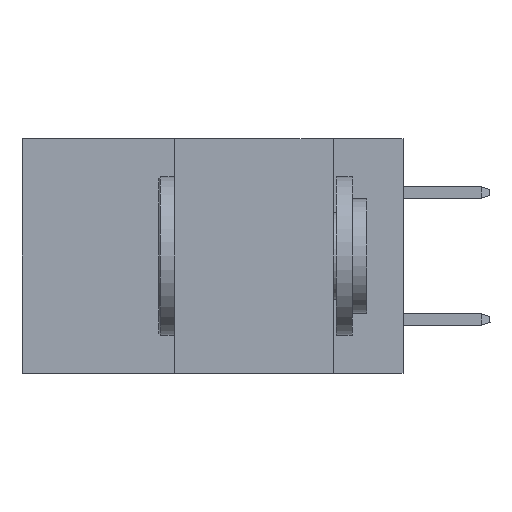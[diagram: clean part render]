
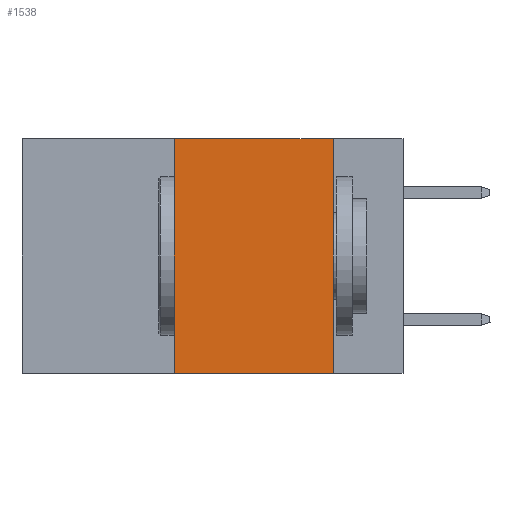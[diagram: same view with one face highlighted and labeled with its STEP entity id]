
A CAD part, left-side view. The second image highlights one B-rep face of the part: STEP entity #1538.
In plain terms, the highlighted planar face has unit normal (-1, 0, 0).
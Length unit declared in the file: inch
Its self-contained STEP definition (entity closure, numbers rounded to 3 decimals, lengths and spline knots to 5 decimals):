
#466 = CARTESIAN_POINT ( 'NONE',  ( 0., 0.11, 0. ) ) ;
#856 = CARTESIAN_POINT ( 'NONE',  ( 0., 0.11, -0.37 ) ) ;
#1538 = ADVANCED_FACE ( 'NONE', ( #15364 ), #13145, .F. ) ;
#1801 = CARTESIAN_POINT ( 'NONE',  ( 0., 0.6, -0.37 ) ) ;
#2632 = EDGE_CURVE ( 'NONE', #18312, #16946, #3755, .T. ) ;
#3384 = CARTESIAN_POINT ( 'NONE',  ( 0., 0.11, 0. ) ) ;
#3755 = LINE ( 'NONE', #5179, #25534 ) ;
#3972 = ORIENTED_EDGE ( 'NONE', *, *, #8624, .F. ) ;
#4328 = DIRECTION ( 'NONE',  ( 0., 0., -1. ) ) ;
#5179 = CARTESIAN_POINT ( 'NONE',  ( 0., 0.6, 0. ) ) ;
#7043 = VECTOR ( 'NONE', #14116, 39.37008 ) ;
#7500 = EDGE_LOOP ( 'NONE', ( #3972, #11106, #10011, #26549 ) ) ;
#8624 = EDGE_CURVE ( 'NONE', #16946, #23303, #17607, .T. ) ;
#10011 = ORIENTED_EDGE ( 'NONE', *, *, #16116, .F. ) ;
#10650 = DIRECTION ( 'NONE',  ( 0., -1., 0. ) ) ;
#11106 = ORIENTED_EDGE ( 'NONE', *, *, #2632, .F. ) ;
#12584 = LINE ( 'NONE', #1801, #18261 ) ;
#13145 = PLANE ( 'NONE',  #22838 ) ;
#13830 = CARTESIAN_POINT ( 'NONE',  ( 0., 0.36, 0. ) ) ;
#14116 = DIRECTION ( 'NONE',  ( 0., 0., 1. ) ) ;
#15099 = DIRECTION ( 'NONE',  ( 1., 0., 0. ) ) ;
#15364 = FACE_OUTER_BOUND ( 'NONE', #7500, .T. ) ;
#15637 = DIRECTION ( 'NONE',  ( 0., 0., -1. ) ) ;
#16116 = EDGE_CURVE ( 'NONE', #26773, #18312, #22406, .T. ) ;
#16946 = VERTEX_POINT ( 'NONE', #3384 ) ;
#17607 = LINE ( 'NONE', #466, #17929 ) ;
#17929 = VECTOR ( 'NONE', #4328, 39.37008 ) ;
#18261 = VECTOR ( 'NONE', #10650, 39.37008 ) ;
#18312 = VERTEX_POINT ( 'NONE', #26356 ) ;
#18567 = DIRECTION ( 'NONE',  ( 0., -1., 0. ) ) ;
#22406 = LINE ( 'NONE', #13830, #7043 ) ;
#22838 = AXIS2_PLACEMENT_3D ( 'NONE', #26151, #15099, #15637 ) ;
#23303 = VERTEX_POINT ( 'NONE', #856 ) ;
#23594 = EDGE_CURVE ( 'NONE', #26773, #23303, #12584, .T. ) ;
#25011 = CARTESIAN_POINT ( 'NONE',  ( 0., 0.36, -0.37 ) ) ;
#25534 = VECTOR ( 'NONE', #18567, 39.37008 ) ;
#26151 = CARTESIAN_POINT ( 'NONE',  ( 0., 0.6, 0. ) ) ;
#26356 = CARTESIAN_POINT ( 'NONE',  ( 0., 0.36, 0. ) ) ;
#26549 = ORIENTED_EDGE ( 'NONE', *, *, #23594, .T. ) ;
#26773 = VERTEX_POINT ( 'NONE', #25011 ) ;
